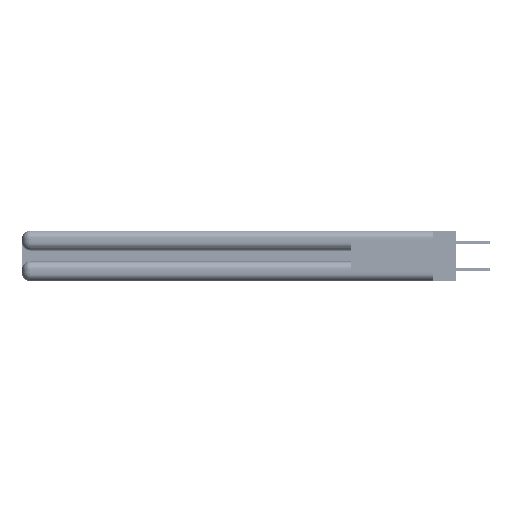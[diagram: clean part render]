
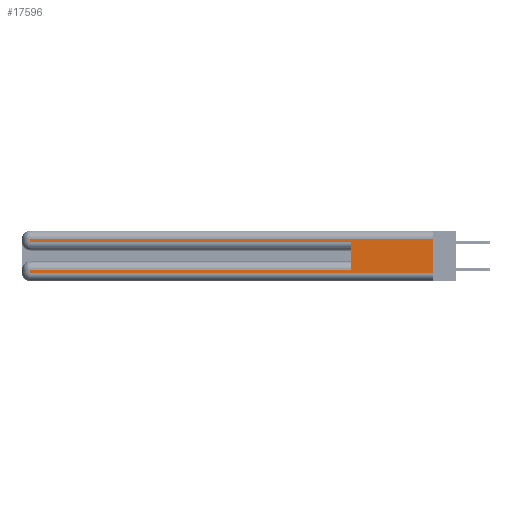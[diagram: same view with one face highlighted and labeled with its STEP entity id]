
A CAD part, left-side view. The second image highlights one B-rep face of the part: STEP entity #17596.
In plain terms, the highlighted planar face has unit normal (-1, 0, 0).
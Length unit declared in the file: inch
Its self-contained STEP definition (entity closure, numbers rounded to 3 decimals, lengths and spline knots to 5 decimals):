
#136 = DIRECTION ( 'NONE',  ( 0., 0., -1. ) ) ;
#795 = LINE ( 'NONE', #53206, #53296 ) ;
#915 = DIRECTION ( 'NONE',  ( 0., 0., -1. ) ) ;
#1041 = EDGE_CURVE ( 'NONE', #5612, #50757, #37979, .T. ) ;
#1062 = AXIS2_PLACEMENT_3D ( 'NONE', #47618, #17867, #915 ) ;
#1194 = EDGE_CURVE ( 'NONE', #21129, #7542, #27824, .T. ) ;
#1806 = CARTESIAN_POINT ( 'NONE',  ( 0., 0.6, 0.285 ) ) ;
#3050 = CARTESIAN_POINT ( 'NONE',  ( 0., 0., 0.085 ) ) ;
#4297 = VECTOR ( 'NONE', #45107, 39.37008 ) ;
#5612 = VERTEX_POINT ( 'NONE', #46406 ) ;
#7272 = EDGE_CURVE ( 'NONE', #45188, #16631, #21488, .T. ) ;
#7542 = VERTEX_POINT ( 'NONE', #22596 ) ;
#8236 = ORIENTED_EDGE ( 'NONE', *, *, #1194, .T. ) ;
#11872 = DIRECTION ( 'NONE',  ( 0., 1., 0. ) ) ;
#11986 = CARTESIAN_POINT ( 'NONE',  ( 0., 0., 0.06 ) ) ;
#12615 = ORIENTED_EDGE ( 'NONE', *, *, #12796, .T. ) ;
#12764 = VECTOR ( 'NONE', #20169, 39.37008 ) ;
#12796 = EDGE_CURVE ( 'NONE', #18262, #21129, #28634, .T. ) ;
#12851 = DIRECTION ( 'NONE',  ( 0., -1., 0. ) ) ;
#12968 = CARTESIAN_POINT ( 'NONE',  ( 0., 2.94, 0.37 ) ) ;
#13552 = PLANE ( 'NONE',  #1062 ) ;
#14029 = LINE ( 'NONE', #27040, #34927 ) ;
#14116 = ORIENTED_EDGE ( 'NONE', *, *, #24474, .F. ) ;
#15662 = CARTESIAN_POINT ( 'NONE',  ( 0., 0., 0.285 ) ) ;
#16631 = VERTEX_POINT ( 'NONE', #1806 ) ;
#16994 = FACE_OUTER_BOUND ( 'NONE', #19567, .T. ) ;
#17274 = ORIENTED_EDGE ( 'NONE', *, *, #1041, .T. ) ;
#17596 = ADVANCED_FACE ( 'NONE', ( #16994 ), #13552, .F. ) ;
#17867 = DIRECTION ( 'NONE',  ( 1., 0., 0. ) ) ;
#18262 = VERTEX_POINT ( 'NONE', #35026 ) ;
#18958 = EDGE_CURVE ( 'NONE', #50757, #45188, #14029, .T. ) ;
#19567 = EDGE_LOOP ( 'NONE', ( #40158, #17274, #48046, #40809, #14116, #12615, #8236, #42498 ) ) ;
#19899 = CARTESIAN_POINT ( 'NONE',  ( 0., 0.6, 0.145 ) ) ;
#20169 = DIRECTION ( 'NONE',  ( 0., -1., 0. ) ) ;
#21129 = VERTEX_POINT ( 'NONE', #55548 ) ;
#21233 = CARTESIAN_POINT ( 'NONE',  ( 0., 0., 0.31 ) ) ;
#21488 = LINE ( 'NONE', #15662, #12764 ) ;
#22461 = VECTOR ( 'NONE', #11872, 39.37008 ) ;
#22493 = LINE ( 'NONE', #19899, #4297 ) ;
#22502 = LINE ( 'NONE', #26024, #32611 ) ;
#22596 = CARTESIAN_POINT ( 'NONE',  ( 0., 2.94, 0.06 ) ) ;
#23112 = VECTOR ( 'NONE', #136, 39.37008 ) ;
#23811 = DIRECTION ( 'NONE',  ( 0., 0., -1. ) ) ;
#24474 = EDGE_CURVE ( 'NONE', #18262, #16631, #22493, .T. ) ;
#26024 = CARTESIAN_POINT ( 'NONE',  ( 0., 0., 0.06 ) ) ;
#27040 = CARTESIAN_POINT ( 'NONE',  ( 0., 2.94, 0.37 ) ) ;
#27824 = LINE ( 'NONE', #12968, #23112 ) ;
#28634 = LINE ( 'NONE', #3050, #42767 ) ;
#32611 = VECTOR ( 'NONE', #12851, 39.37008 ) ;
#34071 = CARTESIAN_POINT ( 'NONE',  ( 0., 2.94, 0.31 ) ) ;
#34579 = VERTEX_POINT ( 'NONE', #11986 ) ;
#34927 = VECTOR ( 'NONE', #40015, 39.37008 ) ;
#35026 = CARTESIAN_POINT ( 'NONE',  ( 0., 0.6, 0.085 ) ) ;
#35520 = EDGE_CURVE ( 'NONE', #7542, #34579, #22502, .T. ) ;
#37018 = EDGE_CURVE ( 'NONE', #5612, #34579, #795, .T. ) ;
#37979 = LINE ( 'NONE', #21233, #22461 ) ;
#40015 = DIRECTION ( 'NONE',  ( 0., 0., -1. ) ) ;
#40158 = ORIENTED_EDGE ( 'NONE', *, *, #37018, .F. ) ;
#40809 = ORIENTED_EDGE ( 'NONE', *, *, #7272, .T. ) ;
#42382 = DIRECTION ( 'NONE',  ( 0., 1., 0. ) ) ;
#42498 = ORIENTED_EDGE ( 'NONE', *, *, #35520, .T. ) ;
#42767 = VECTOR ( 'NONE', #42382, 39.37008 ) ;
#45107 = DIRECTION ( 'NONE',  ( 0., 0., 1. ) ) ;
#45188 = VERTEX_POINT ( 'NONE', #49405 ) ;
#46406 = CARTESIAN_POINT ( 'NONE',  ( 0., 0., 0.31 ) ) ;
#47618 = CARTESIAN_POINT ( 'NONE',  ( 0., 0., 0.37 ) ) ;
#48046 = ORIENTED_EDGE ( 'NONE', *, *, #18958, .T. ) ;
#49405 = CARTESIAN_POINT ( 'NONE',  ( 0., 2.94, 0.285 ) ) ;
#50757 = VERTEX_POINT ( 'NONE', #34071 ) ;
#53206 = CARTESIAN_POINT ( 'NONE',  ( 0., 0., 0.37 ) ) ;
#53296 = VECTOR ( 'NONE', #23811, 39.37008 ) ;
#55548 = CARTESIAN_POINT ( 'NONE',  ( 0., 2.94, 0.085 ) ) ;
